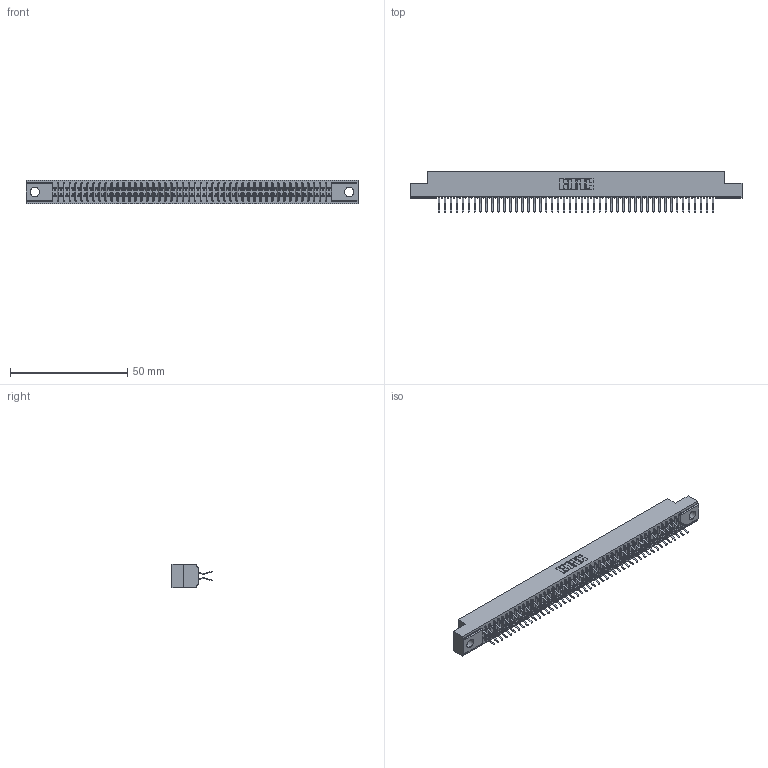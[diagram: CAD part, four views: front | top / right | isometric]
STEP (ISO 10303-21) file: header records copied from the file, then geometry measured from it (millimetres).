
FILE_DESCRIPTION (( 'STEP AP203' ), '1' );
FILE_NAME ('391-094-556-204.STEP', '2018-08-09T18:22:18', ( '' ), ( '' ), 'SwSTEP 2.0', 'SolidWorks 2016', '' );
FILE_SCHEMA (( 'CONFIG_CONTROL_DESIGN' ));
Length unit declared in the file: inch
Products named in the file (3): 341-292-001_341-292-156; 391-094-556-204; 341 Part_.156 (3.96) Dia Mounting Holes
Assembly tree (95 placements, depth 2):
  391-094-556-204
    341 Part_.156 (3.96) Dia Mounting Holes
    341-292-001_341-292-156  x94
Bounding box: 141.6 x 17.07 x 10.16 mm (x, y, z)
Volume: 10385.2 mm3; surface area: 18704.1 mm2
Topology: 95 solids, 95 shells, 6710 faces, 19481 edges, 12638 vertices
Faces by surface type: plane 3842, cylinder 2680, sphere 96, torus 92
Entity records: 56772 total; most frequent: CARTESIAN_POINT 9443, ORIENTED_EDGE 9382, DIRECTION 9157, EDGE_CURVE 4691, LINE 3797, VECTOR 3797, VERTEX_POINT 2966, AXIS2_PLACEMENT_3D 2680
